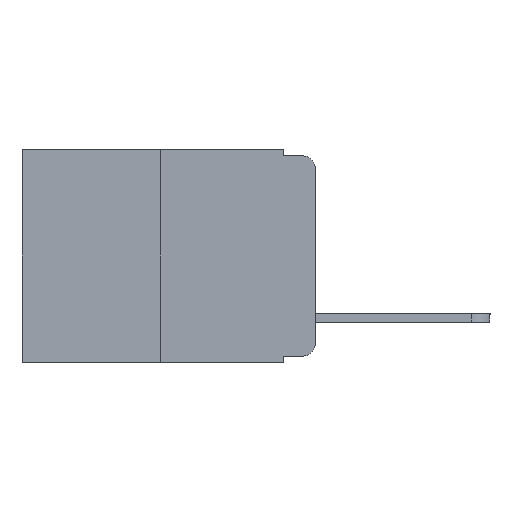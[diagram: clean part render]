
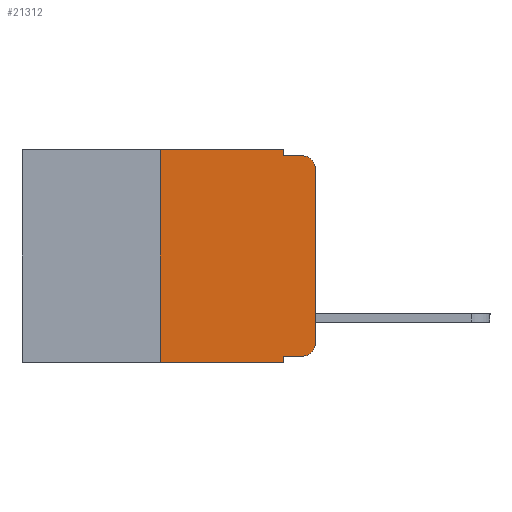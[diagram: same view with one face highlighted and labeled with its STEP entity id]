
A CAD part, left-side view. The second image highlights one B-rep face of the part: STEP entity #21312.
In plain terms, the highlighted planar face has unit normal (-1, 0, 0).
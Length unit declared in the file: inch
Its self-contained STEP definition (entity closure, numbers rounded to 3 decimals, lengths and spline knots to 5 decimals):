
#40 = DIRECTION ( 'NONE',  ( 0., 0., -1. ) ) ;
#719 = ORIENTED_EDGE ( 'NONE', *, *, #8723, .T. ) ;
#897 = VECTOR ( 'NONE', #1244, 39.37008 ) ;
#898 = DIRECTION ( 'NONE',  ( 0., 0., -1. ) ) ;
#908 = VERTEX_POINT ( 'NONE', #18999 ) ;
#946 = EDGE_CURVE ( 'NONE', #7130, #3794, #7122, .T. ) ;
#1027 = CARTESIAN_POINT ( 'NONE',  ( 0., 0.473, 0. ) ) ;
#1244 = DIRECTION ( 'NONE',  ( 0., -1., 0. ) ) ;
#1694 = CARTESIAN_POINT ( 'NONE',  ( 0., 0.051, 0. ) ) ;
#1881 = DIRECTION ( 'NONE',  ( 0., -1., 0. ) ) ;
#2085 = EDGE_CURVE ( 'NONE', #12441, #16989, #9640, .T. ) ;
#2709 = DIRECTION ( 'NONE',  ( 0., 0., -1. ) ) ;
#3135 = CARTESIAN_POINT ( 'NONE',  ( 0., 0., -0.313 ) ) ;
#3380 = VECTOR ( 'NONE', #1881, 39.37008 ) ;
#3794 = VERTEX_POINT ( 'NONE', #17935 ) ;
#4295 = EDGE_CURVE ( 'NONE', #8959, #4735, #19752, .T. ) ;
#4309 = LINE ( 'NONE', #14804, #21443 ) ;
#4330 = CARTESIAN_POINT ( 'NONE',  ( 0., 0.02, -0.333 ) ) ;
#4409 = VECTOR ( 'NONE', #9380, 39.37008 ) ;
#4454 = CARTESIAN_POINT ( 'NONE',  ( 0., 0., -0.03 ) ) ;
#4622 = CIRCLE ( 'NONE', #12422, 0.02 ) ;
#4735 = VERTEX_POINT ( 'NONE', #8566 ) ;
#5770 = ORIENTED_EDGE ( 'NONE', *, *, #946, .F. ) ;
#6541 = EDGE_CURVE ( 'NONE', #4735, #908, #14334, .T. ) ;
#7122 = LINE ( 'NONE', #1694, #19374 ) ;
#7130 = VERTEX_POINT ( 'NONE', #20813 ) ;
#7510 = CARTESIAN_POINT ( 'NONE',  ( 0., 0.051, 0. ) ) ;
#7626 = EDGE_CURVE ( 'NONE', #12296, #908, #4622, .T. ) ;
#7730 = CARTESIAN_POINT ( 'NONE',  ( 0., 0.051, -0.01 ) ) ;
#7783 = LINE ( 'NONE', #13468, #3380 ) ;
#7833 = ORIENTED_EDGE ( 'NONE', *, *, #4295, .F. ) ;
#8255 = VECTOR ( 'NONE', #19970, 39.37008 ) ;
#8566 = CARTESIAN_POINT ( 'NONE',  ( 0., 0.051, -0.01 ) ) ;
#8685 = DIRECTION ( 'NONE',  ( 0., 0., -1. ) ) ;
#8723 = EDGE_CURVE ( 'NONE', #11294, #12296, #4309, .T. ) ;
#8757 = CARTESIAN_POINT ( 'NONE',  ( 0., 0.051, 0. ) ) ;
#8959 = VERTEX_POINT ( 'NONE', #8757 ) ;
#9108 = VECTOR ( 'NONE', #14549, 39.37008 ) ;
#9380 = DIRECTION ( 'NONE',  ( 0., -1., 0. ) ) ;
#9640 = LINE ( 'NONE', #13718, #9108 ) ;
#9719 = LINE ( 'NONE', #21141, #897 ) ;
#9959 = CARTESIAN_POINT ( 'NONE',  ( 0., 0.473, -0.343 ) ) ;
#10045 = DIRECTION ( 'NONE',  ( -1., 0., 0. ) ) ;
#10818 = DIRECTION ( 'NONE',  ( -1., 0., 0. ) ) ;
#11294 = VERTEX_POINT ( 'NONE', #3135 ) ;
#11806 = FACE_OUTER_BOUND ( 'NONE', #15011, .T. ) ;
#11908 = AXIS2_PLACEMENT_3D ( 'NONE', #1027, #12637, #2709 ) ;
#11934 = EDGE_CURVE ( 'NONE', #16989, #8959, #7783, .T. ) ;
#11943 = ORIENTED_EDGE ( 'NONE', *, *, #7626, .T. ) ;
#12136 = ORIENTED_EDGE ( 'NONE', *, *, #2085, .F. ) ;
#12296 = VERTEX_POINT ( 'NONE', #4454 ) ;
#12422 = AXIS2_PLACEMENT_3D ( 'NONE', #20797, #10818, #898 ) ;
#12441 = VERTEX_POINT ( 'NONE', #21355 ) ;
#12504 = DIRECTION ( 'NONE',  ( 0., 0., -1. ) ) ;
#12637 = DIRECTION ( 'NONE',  ( 1., 0., 0. ) ) ;
#12662 = LINE ( 'NONE', #9959, #8255 ) ;
#13141 = DIRECTION ( 'NONE',  ( 0., 0., 1. ) ) ;
#13468 = CARTESIAN_POINT ( 'NONE',  ( 0., 0.473, 0. ) ) ;
#13718 = CARTESIAN_POINT ( 'NONE',  ( 0., 0.25, 0. ) ) ;
#14296 = ORIENTED_EDGE ( 'NONE', *, *, #15091, .T. ) ;
#14334 = LINE ( 'NONE', #7730, #4409 ) ;
#14549 = DIRECTION ( 'NONE',  ( 0., 0., 1. ) ) ;
#14710 = ORIENTED_EDGE ( 'NONE', *, *, #11934, .F. ) ;
#14804 = CARTESIAN_POINT ( 'NONE',  ( 0., 0., 0. ) ) ;
#14871 = CIRCLE ( 'NONE', #20273, 0.02 ) ;
#15011 = EDGE_LOOP ( 'NONE', ( #719, #11943, #20082, #7833, #14710, #12136, #14296, #5770, #15218, #19407 ) ) ;
#15091 = EDGE_CURVE ( 'NONE', #12441, #3794, #12662, .T. ) ;
#15218 = ORIENTED_EDGE ( 'NONE', *, *, #21393, .T. ) ;
#15377 = VECTOR ( 'NONE', #12504, 39.37008 ) ;
#16021 = PLANE ( 'NONE',  #11908 ) ;
#16989 = VERTEX_POINT ( 'NONE', #18557 ) ;
#17935 = CARTESIAN_POINT ( 'NONE',  ( 0., 0.051, -0.343 ) ) ;
#18557 = CARTESIAN_POINT ( 'NONE',  ( 0., 0.25, 0. ) ) ;
#18800 = VERTEX_POINT ( 'NONE', #4330 ) ;
#18999 = CARTESIAN_POINT ( 'NONE',  ( 0., 0.02, -0.01 ) ) ;
#19374 = VECTOR ( 'NONE', #8685, 39.37008 ) ;
#19407 = ORIENTED_EDGE ( 'NONE', *, *, #20304, .T. ) ;
#19752 = LINE ( 'NONE', #7510, #15377 ) ;
#19970 = DIRECTION ( 'NONE',  ( 0., -1., 0. ) ) ;
#20056 = CARTESIAN_POINT ( 'NONE',  ( 0., 0.02, -0.313 ) ) ;
#20082 = ORIENTED_EDGE ( 'NONE', *, *, #6541, .F. ) ;
#20273 = AXIS2_PLACEMENT_3D ( 'NONE', #20056, #10045, #40 ) ;
#20304 = EDGE_CURVE ( 'NONE', #18800, #11294, #14871, .T. ) ;
#20797 = CARTESIAN_POINT ( 'NONE',  ( 0., 0.02, -0.03 ) ) ;
#20813 = CARTESIAN_POINT ( 'NONE',  ( 0., 0.051, -0.333 ) ) ;
#21141 = CARTESIAN_POINT ( 'NONE',  ( 0., 0.051, -0.333 ) ) ;
#21312 = ADVANCED_FACE ( 'NONE', ( #11806 ), #16021, .F. ) ;
#21355 = CARTESIAN_POINT ( 'NONE',  ( 0., 0.25, -0.343 ) ) ;
#21393 = EDGE_CURVE ( 'NONE', #7130, #18800, #9719, .T. ) ;
#21443 = VECTOR ( 'NONE', #13141, 39.37008 ) ;
